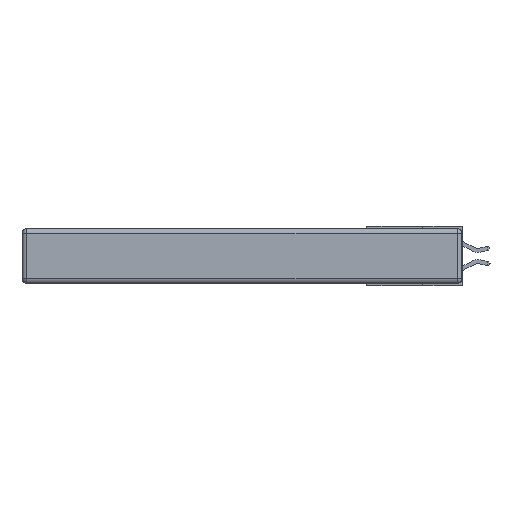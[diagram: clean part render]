
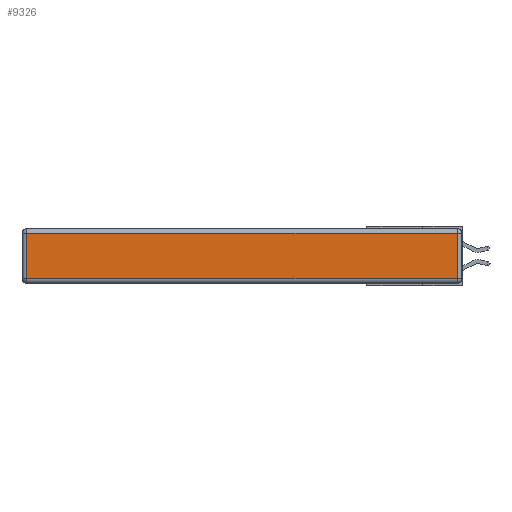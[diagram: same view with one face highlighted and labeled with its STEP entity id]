
A CAD part, left-side view. The second image highlights one B-rep face of the part: STEP entity #9326.
In plain terms, the highlighted planar face has unit normal (-1, 0, 0).
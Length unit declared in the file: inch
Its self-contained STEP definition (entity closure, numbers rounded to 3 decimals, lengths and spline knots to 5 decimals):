
#229 = CARTESIAN_POINT ( 'NONE',  ( 0., 2.75, -0.03 ) ) ;
#360 = ORIENTED_EDGE ( 'NONE', *, *, #18047, .T. ) ;
#724 = DIRECTION ( 'NONE',  ( 0., 0., 1. ) ) ;
#861 = VERTEX_POINT ( 'NONE', #12735 ) ;
#1187 = PLANE ( 'NONE',  #16862 ) ;
#1411 = EDGE_CURVE ( 'NONE', #14461, #10138, #2025, .T. ) ;
#1466 = EDGE_LOOP ( 'NONE', ( #11533, #360, #8950, #18601 ) ) ;
#1788 = DIRECTION ( 'NONE',  ( 0., 0., -1. ) ) ;
#1833 = LINE ( 'NONE', #4586, #11815 ) ;
#2025 = LINE ( 'NONE', #229, #7927 ) ;
#3173 = EDGE_CURVE ( 'NONE', #861, #5505, #12368, .T. ) ;
#4205 = CARTESIAN_POINT ( 'NONE',  ( 0., 0.03, -0.313 ) ) ;
#4445 = LINE ( 'NONE', #6305, #16652 ) ;
#4586 = CARTESIAN_POINT ( 'NONE',  ( 0., 2.72, -0.343 ) ) ;
#4696 = CARTESIAN_POINT ( 'NONE',  ( 0., 0., -0.313 ) ) ;
#5505 = VERTEX_POINT ( 'NONE', #4205 ) ;
#6305 = CARTESIAN_POINT ( 'NONE',  ( 0., 0.03, -0.343 ) ) ;
#6542 = EDGE_CURVE ( 'NONE', #10138, #861, #1833, .T. ) ;
#7927 = VECTOR ( 'NONE', #10375, 39.37008 ) ;
#8046 = CARTESIAN_POINT ( 'NONE',  ( 0., 0.03, -0.03 ) ) ;
#8586 = DIRECTION ( 'NONE',  ( 0., 0., 1. ) ) ;
#8950 = ORIENTED_EDGE ( 'NONE', *, *, #1411, .T. ) ;
#9326 = ADVANCED_FACE ( 'NONE', ( #15813 ), #1187, .T. ) ;
#10138 = VERTEX_POINT ( 'NONE', #13211 ) ;
#10375 = DIRECTION ( 'NONE',  ( 0., 1., 0. ) ) ;
#11432 = DIRECTION ( 'NONE',  ( -1., 0., 0. ) ) ;
#11533 = ORIENTED_EDGE ( 'NONE', *, *, #3173, .T. ) ;
#11815 = VECTOR ( 'NONE', #1788, 39.37008 ) ;
#12368 = LINE ( 'NONE', #4696, #18032 ) ;
#12735 = CARTESIAN_POINT ( 'NONE',  ( 0., 2.72, -0.313 ) ) ;
#13211 = CARTESIAN_POINT ( 'NONE',  ( 0., 2.72, -0.03 ) ) ;
#14461 = VERTEX_POINT ( 'NONE', #8046 ) ;
#15813 = FACE_OUTER_BOUND ( 'NONE', #1466, .T. ) ;
#16652 = VECTOR ( 'NONE', #724, 39.37008 ) ;
#16862 = AXIS2_PLACEMENT_3D ( 'NONE', #18654, #11432, #8586 ) ;
#18032 = VECTOR ( 'NONE', #18109, 39.37008 ) ;
#18047 = EDGE_CURVE ( 'NONE', #5505, #14461, #4445, .T. ) ;
#18109 = DIRECTION ( 'NONE',  ( 0., -1., 0. ) ) ;
#18601 = ORIENTED_EDGE ( 'NONE', *, *, #6542, .T. ) ;
#18654 = CARTESIAN_POINT ( 'NONE',  ( 0., 0., -0.343 ) ) ;
